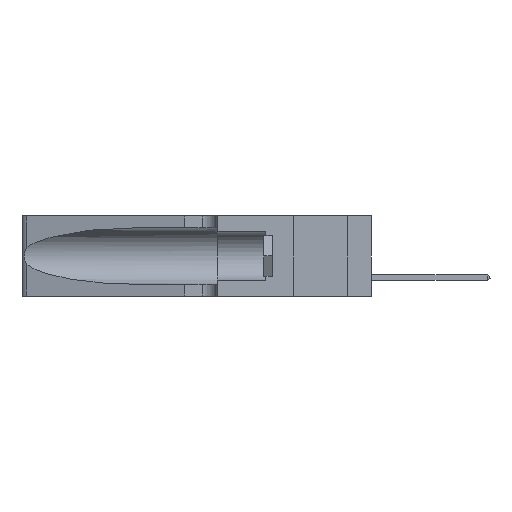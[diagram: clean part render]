
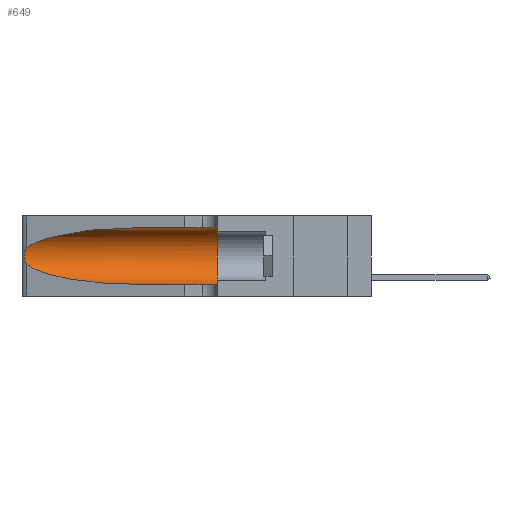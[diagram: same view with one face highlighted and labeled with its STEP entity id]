
A CAD part, left-side view. The second image highlights one B-rep face of the part: STEP entity #649.
In plain terms, the highlighted cylindrical face has radius 3.308 mm (diameter 6.617 mm), a partial arc.
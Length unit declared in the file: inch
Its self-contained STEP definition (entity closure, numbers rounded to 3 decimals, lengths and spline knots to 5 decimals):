
#649 = ADVANCED_FACE ( 'NONE', ( #37930 ), #25497, .F. ) ;
#1272 = CIRCLE ( 'NONE', #37296, 0.13025 ) ;
#1488 = VERTEX_POINT ( 'NONE', #14714 ) ;
#1554 = CARTESIAN_POINT ( 'NONE',  ( 0.25555, 1.22993, 0.14849 ) ) ;
#1958 = ORIENTED_EDGE ( 'NONE', *, *, #10499, .T. ) ;
#1980 = ORIENTED_EDGE ( 'NONE', *, *, #19629, .F. ) ;
#2069 = CARTESIAN_POINT ( 'NONE',  ( 0.25787, 1.23484, 0.2124 ) ) ;
#3987 = CARTESIAN_POINT ( 'NONE',  ( 0.2373, 1.15595, 0.28018 ) ) ;
#4536 = CARTESIAN_POINT ( 'NONE',  ( 0.25487, 1.22718, 0.14631 ) ) ;
#5059 = CARTESIAN_POINT ( 'NONE',  ( 0.26018, 1.23835, 0.19895 ) ) ;
#5068 = VECTOR ( 'NONE', #23253, 39.37008 ) ;
#7048 = ORIENTED_EDGE ( 'NONE', *, *, #27979, .F. ) ;
#7796 =( BOUNDED_CURVE ( )  B_SPLINE_CURVE ( 3, ( #22241, #21531, #3987, #36625 ),
 .UNSPECIFIED., .F., .F. ) 
 B_SPLINE_CURVE_WITH_KNOTS ( ( 4, 4 ),
 ( 1.5708, 2.84003 ),
 .UNSPECIFIED. ) 
 CURVE ( )  GEOMETRIC_REPRESENTATION_ITEM ( )  RATIONAL_B_SPLINE_CURVE ( ( 1., 0.87, 0.87, 1. ) ) 
 REPRESENTATION_ITEM ( '' )  );
#8321 = CARTESIAN_POINT ( 'NONE',  ( 0.18966, 0.96281, 0.05475 ) ) ;
#8456 = VERTEX_POINT ( 'NONE', #17788 ) ;
#9207 = EDGE_LOOP ( 'NONE', ( #30788, #32503, #1958, #34661, #7048, #1980 ) ) ;
#9588 = EDGE_CURVE ( 'NONE', #8456, #14039, #7796, .T. ) ;
#10301 = CARTESIAN_POINT ( 'NONE',  ( 0.26075, 1.23896, 0.178 ) ) ;
#10499 = EDGE_CURVE ( 'NONE', #1488, #11707, #37337, .T. ) ;
#11232 = CARTESIAN_POINT ( 'NONE',  ( 0.1305, 0.72297, 0.05475 ) ) ;
#11707 = VERTEX_POINT ( 'NONE', #31249 ) ;
#12157 = VECTOR ( 'NONE', #20093, 39.37008 ) ;
#12956 = DIRECTION ( 'NONE',  ( 0., 0., -1. ) ) ;
#13266 = CARTESIAN_POINT ( 'NONE',  ( 0.25856, 1.23593, 0.16098 ) ) ;
#13412 = CARTESIAN_POINT ( 'NONE',  ( 0.25555, 1.22994, 0.2215 ) ) ;
#14039 = VERTEX_POINT ( 'NONE', #19555 ) ;
#14714 = CARTESIAN_POINT ( 'NONE',  ( 0.25487, 1.22718, 0.14631 ) ) ;
#15415 = LINE ( 'NONE', #34527, #12157 ) ;
#16281 = CARTESIAN_POINT ( 'NONE',  ( 0.25789, 1.23486, 0.15765 ) ) ;
#16571 = CARTESIAN_POINT ( 'NONE',  ( 0.1305, 0.35, 0.185 ) ) ;
#17788 = CARTESIAN_POINT ( 'NONE',  ( 0.1305, 0.72297, 0.31525 ) ) ;
#19219 = CARTESIAN_POINT ( 'NONE',  ( 0.25487, 1.22718, 0.22369 ) ) ;
#19555 = CARTESIAN_POINT ( 'NONE',  ( 0.25487, 1.22718, 0.22369 ) ) ;
#19629 = EDGE_CURVE ( 'NONE', #8456, #27731, #15415, .T. ) ;
#20093 = DIRECTION ( 'NONE',  ( 0., -1., 0. ) ) ;
#20274 = CARTESIAN_POINT ( 'NONE',  ( 0.1305, 1.61858, 0.05475 ) ) ;
#20503 = VERTEX_POINT ( 'NONE', #22876 ) ;
#21531 = CARTESIAN_POINT ( 'NONE',  ( 0.18966, 0.96281, 0.31525 ) ) ;
#22241 = CARTESIAN_POINT ( 'NONE',  ( 0.1305, 0.72297, 0.31525 ) ) ;
#22289 = EDGE_CURVE ( 'NONE', #11707, #20503, #23956, .T. ) ;
#22876 = CARTESIAN_POINT ( 'NONE',  ( 0.1305, 0.35, 0.05475 ) ) ;
#22880 = EDGE_CURVE ( 'NONE', #14039, #1488, #23657, .T. ) ;
#23032 = CARTESIAN_POINT ( 'NONE',  ( 0.2373, 1.15595, 0.08982 ) ) ;
#23253 = DIRECTION ( 'NONE',  ( 0., -1., 0. ) ) ;
#23657 = B_SPLINE_CURVE_WITH_KNOTS ( 'NONE', 3,
 ( #19219, #13412, #34456, #2069, #33944, #5059, #25719, #10301, #30982, #13266, #16281, #36887, #1554, #4536 ),
 .UNSPECIFIED., .F., .F.,
 ( 4, 2, 2, 2, 2, 2, 4 ),
 ( 0., 0.00027, 0.00053, 0.00107, 0.0016, 0.00187, 0.00214 ),
 .UNSPECIFIED. ) ;
#23956 = LINE ( 'NONE', #20274, #5068 ) ;
#25497 = CYLINDRICAL_SURFACE ( 'NONE', #34344, 0.13025 ) ;
#25625 = DIRECTION ( 'NONE',  ( 0., 0., 1. ) ) ;
#25719 = CARTESIAN_POINT ( 'NONE',  ( 0.26075, 1.23896, 0.19203 ) ) ;
#26132 = CARTESIAN_POINT ( 'NONE',  ( 0.25487, 1.22718, 0.14631 ) ) ;
#27731 = VERTEX_POINT ( 'NONE', #36418 ) ;
#27979 = EDGE_CURVE ( 'NONE', #27731, #20503, #1272, .T. ) ;
#30147 = CARTESIAN_POINT ( 'NONE',  ( 0.1305, 1.61858, 0.185 ) ) ;
#30667 = DIRECTION ( 'NONE',  ( 0., -1., 0. ) ) ;
#30788 = ORIENTED_EDGE ( 'NONE', *, *, #9588, .T. ) ;
#30982 = CARTESIAN_POINT ( 'NONE',  ( 0.26017, 1.23833, 0.17102 ) ) ;
#31249 = CARTESIAN_POINT ( 'NONE',  ( 0.1305, 0.72297, 0.05475 ) ) ;
#31401 = DIRECTION ( 'NONE',  ( 0., 1., 0. ) ) ;
#32503 = ORIENTED_EDGE ( 'NONE', *, *, #22880, .T. ) ;
#33944 = CARTESIAN_POINT ( 'NONE',  ( 0.25854, 1.2359, 0.20912 ) ) ;
#34344 = AXIS2_PLACEMENT_3D ( 'NONE', #30147, #30667, #12956 ) ;
#34456 = CARTESIAN_POINT ( 'NONE',  ( 0.25639, 1.23184, 0.21858 ) ) ;
#34527 = CARTESIAN_POINT ( 'NONE',  ( 0.1305, 1.61858, 0.31525 ) ) ;
#34661 = ORIENTED_EDGE ( 'NONE', *, *, #22289, .T. ) ;
#36418 = CARTESIAN_POINT ( 'NONE',  ( 0.1305, 0.35, 0.31525 ) ) ;
#36625 = CARTESIAN_POINT ( 'NONE',  ( 0.25487, 1.22718, 0.22369 ) ) ;
#36887 = CARTESIAN_POINT ( 'NONE',  ( 0.25639, 1.23186, 0.15144 ) ) ;
#37296 = AXIS2_PLACEMENT_3D ( 'NONE', #16571, #31401, #25625 ) ;
#37337 =( BOUNDED_CURVE ( )  B_SPLINE_CURVE ( 3, ( #26132, #23032, #8321, #11232 ),
 .UNSPECIFIED., .F., .T. ) 
 B_SPLINE_CURVE_WITH_KNOTS ( ( 4, 4 ),
 ( 3.44316, 4.71239 ),
 .UNSPECIFIED. ) 
 CURVE ( )  GEOMETRIC_REPRESENTATION_ITEM ( )  RATIONAL_B_SPLINE_CURVE ( ( 1., 0.87, 0.87, 1. ) ) 
 REPRESENTATION_ITEM ( '' )  );
#37930 = FACE_OUTER_BOUND ( 'NONE', #9207, .T. ) ;
